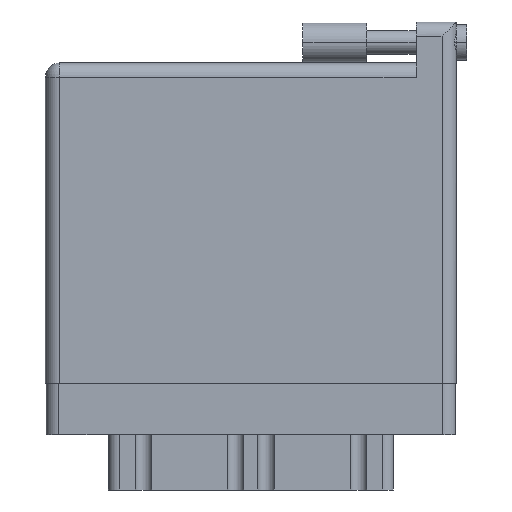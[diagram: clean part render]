
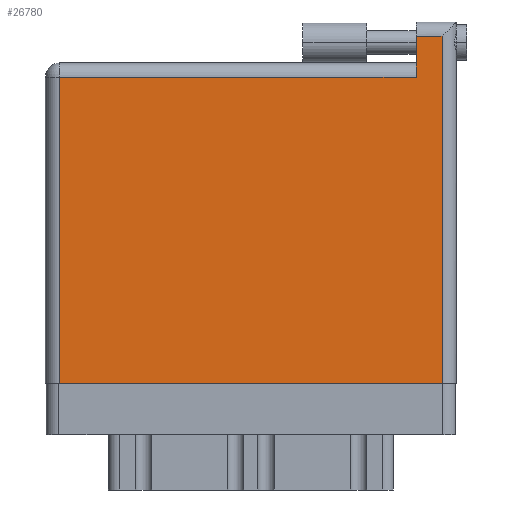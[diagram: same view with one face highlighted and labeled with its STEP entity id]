
A CAD part, front view. The second image highlights one B-rep face of the part: STEP entity #26780.
In plain terms, the highlighted face is planar.
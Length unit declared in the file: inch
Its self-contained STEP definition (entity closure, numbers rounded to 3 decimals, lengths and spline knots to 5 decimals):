
#406 = CARTESIAN_POINT ( 'NONE',  ( 0., 1.696, 0. ) ) ;
#914 = DIRECTION ( 'NONE',  ( -1., 0., 0. ) ) ;
#1498 = VERTEX_POINT ( 'NONE', #13655 ) ;
#2394 = CARTESIAN_POINT ( 'NONE',  ( 0.07, 0., 0. ) ) ;
#2916 = ORIENTED_EDGE ( 'NONE', *, *, #19366, .T. ) ;
#3550 = DIRECTION ( 'NONE',  ( -1., 0., 0. ) ) ;
#5629 = DIRECTION ( 'NONE',  ( 0., 0., -1. ) ) ;
#5944 = VERTEX_POINT ( 'NONE', #2394 ) ;
#6331 = VECTOR ( 'NONE', #29967, 39.37008 ) ;
#7081 = ORIENTED_EDGE ( 'NONE', *, *, #7243, .T. ) ;
#7202 = CARTESIAN_POINT ( 'NONE',  ( 1.811, 1.696, 0. ) ) ;
#7237 = LINE ( 'NONE', #34010, #6331 ) ;
#7243 = EDGE_CURVE ( 'NONE', #23220, #24630, #7237, .T. ) ;
#7581 = VERTEX_POINT ( 'NONE', #7202 ) ;
#8561 = VECTOR ( 'NONE', #30953, 39.37008 ) ;
#8629 = EDGE_CURVE ( 'NONE', #24630, #7581, #24910, .T. ) ;
#9315 = EDGE_LOOP ( 'NONE', ( #19694, #7081, #34247, #26853, #2916, #24268 ) ) ;
#9317 = LINE ( 'NONE', #20156, #26356 ) ;
#10558 = VECTOR ( 'NONE', #32625, 39.37008 ) ;
#10702 = DIRECTION ( 'NONE',  ( -1., 0., 0. ) ) ;
#12028 = AXIS2_PLACEMENT_3D ( 'NONE', #19263, #5629, #10702 ) ;
#12232 = LINE ( 'NONE', #33583, #8561 ) ;
#12550 = EDGE_CURVE ( 'NONE', #5944, #23220, #12232, .T. ) ;
#13334 = FACE_OUTER_BOUND ( 'NONE', #9315, .T. ) ;
#13655 = CARTESIAN_POINT ( 'NONE',  ( 1.811, 1.496, 0. ) ) ;
#16355 = VECTOR ( 'NONE', #22684, 39.37008 ) ;
#16532 = LINE ( 'NONE', #19492, #10558 ) ;
#16620 = VECTOR ( 'NONE', #914, 39.37008 ) ;
#19263 = CARTESIAN_POINT ( 'NONE',  ( 0., 1.566, 0. ) ) ;
#19366 = EDGE_CURVE ( 'NONE', #1498, #29095, #9317, .T. ) ;
#19492 = CARTESIAN_POINT ( 'NONE',  ( 1.811, 1.766, 0. ) ) ;
#19694 = ORIENTED_EDGE ( 'NONE', *, *, #12550, .T. ) ;
#20156 = CARTESIAN_POINT ( 'NONE',  ( 0., 1.496, 0. ) ) ;
#22684 = DIRECTION ( 'NONE',  ( 0., -1., 0. ) ) ;
#23220 = VERTEX_POINT ( 'NONE', #31147 ) ;
#24023 = PLANE ( 'NONE',  #12028 ) ;
#24048 = EDGE_CURVE ( 'NONE', #29095, #5944, #27754, .T. ) ;
#24268 = ORIENTED_EDGE ( 'NONE', *, *, #24048, .T. ) ;
#24630 = VERTEX_POINT ( 'NONE', #27461 ) ;
#24910 = LINE ( 'NONE', #406, #16620 ) ;
#25814 = CARTESIAN_POINT ( 'NONE',  ( 0.07, 0., 0. ) ) ;
#26356 = VECTOR ( 'NONE', #3550, 39.37008 ) ;
#26780 = ADVANCED_FACE ( 'NONE', ( #13334 ), #24023, .F. ) ;
#26853 = ORIENTED_EDGE ( 'NONE', *, *, #30587, .T. ) ;
#27461 = CARTESIAN_POINT ( 'NONE',  ( 1.938, 1.696, 0. ) ) ;
#27754 = LINE ( 'NONE', #25814, #16355 ) ;
#29095 = VERTEX_POINT ( 'NONE', #30894 ) ;
#29967 = DIRECTION ( 'NONE',  ( 0., 1., 0. ) ) ;
#30587 = EDGE_CURVE ( 'NONE', #7581, #1498, #16532, .T. ) ;
#30894 = CARTESIAN_POINT ( 'NONE',  ( 0.07, 1.496, 0. ) ) ;
#30953 = DIRECTION ( 'NONE',  ( 1., 0., 0. ) ) ;
#31147 = CARTESIAN_POINT ( 'NONE',  ( 1.938, 0., 0. ) ) ;
#32625 = DIRECTION ( 'NONE',  ( 0., -1., 0. ) ) ;
#33583 = CARTESIAN_POINT ( 'NONE',  ( 0., 0., 0. ) ) ;
#34010 = CARTESIAN_POINT ( 'NONE',  ( 1.938, 1.766, 0. ) ) ;
#34247 = ORIENTED_EDGE ( 'NONE', *, *, #8629, .T. ) ;
